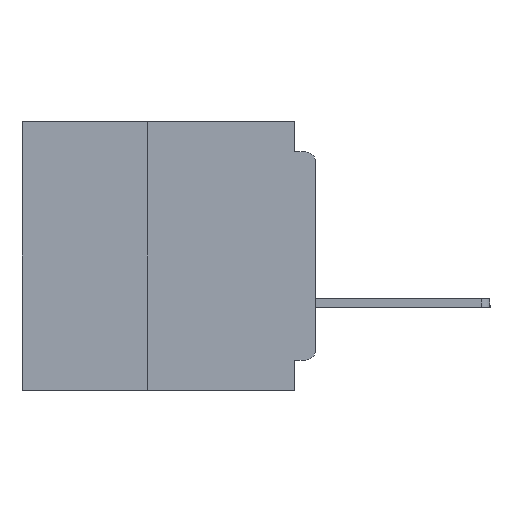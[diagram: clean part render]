
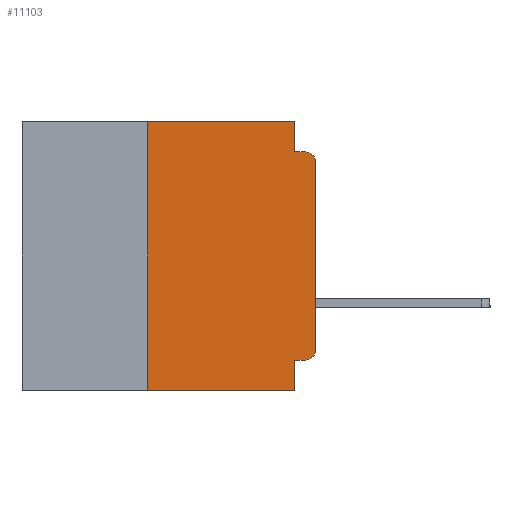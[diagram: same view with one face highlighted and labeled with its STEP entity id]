
A CAD part, left-side view. The second image highlights one B-rep face of the part: STEP entity #11103.
In plain terms, the highlighted planar face has unit normal (-1, 0, 0).
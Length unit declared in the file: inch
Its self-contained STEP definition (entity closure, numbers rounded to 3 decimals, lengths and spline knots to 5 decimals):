
#65 = CARTESIAN_POINT ( 'NONE',  ( 0., 0.031, -0.4 ) ) ;
#816 = AXIS2_PLACEMENT_3D ( 'NONE', #25689, #5339, #28968 ) ;
#1196 = EDGE_CURVE ( 'NONE', #15141, #7626, #9564, .T. ) ;
#1341 = VECTOR ( 'NONE', #21800, 39.37008 ) ;
#3353 = CIRCLE ( 'NONE', #23624, 0.015 ) ;
#3932 = VERTEX_POINT ( 'NONE', #65 ) ;
#4662 = CARTESIAN_POINT ( 'NONE',  ( 0., 0.25, -0.4 ) ) ;
#4825 = FACE_OUTER_BOUND ( 'NONE', #36976, .T. ) ;
#5259 = CARTESIAN_POINT ( 'NONE',  ( 0., 0., 0. ) ) ;
#5339 = DIRECTION ( 'NONE',  ( 1., 0., 0. ) ) ;
#5525 = VECTOR ( 'NONE', #8779, 39.37008 ) ;
#5892 = DIRECTION ( 'NONE',  ( 0., 0., -1. ) ) ;
#6065 = CARTESIAN_POINT ( 'NONE',  ( 0., 0.015, -0.355 ) ) ;
#7496 = CARTESIAN_POINT ( 'NONE',  ( 0., 0.437, 0. ) ) ;
#7626 = VERTEX_POINT ( 'NONE', #27727 ) ;
#8749 = DIRECTION ( 'NONE',  ( 0., 0., 1. ) ) ;
#8779 = DIRECTION ( 'NONE',  ( 0., 0., 1. ) ) ;
#8889 = EDGE_CURVE ( 'NONE', #15141, #21092, #3353, .T. ) ;
#9010 = VERTEX_POINT ( 'NONE', #21100 ) ;
#9564 = LINE ( 'NONE', #28296, #35123 ) ;
#10329 = VERTEX_POINT ( 'NONE', #4662 ) ;
#10991 = DIRECTION ( 'NONE',  ( 0., -1., 0. ) ) ;
#11103 = ADVANCED_FACE ( 'NONE', ( #4825 ), #35420, .F. ) ;
#11639 = LINE ( 'NONE', #5259, #19604 ) ;
#12084 = ORIENTED_EDGE ( 'NONE', *, *, #42866, .F. ) ;
#12362 = CARTESIAN_POINT ( 'NONE',  ( 0., 0., -0.06 ) ) ;
#13687 = EDGE_CURVE ( 'NONE', #32011, #25730, #17010, .T. ) ;
#13967 = EDGE_CURVE ( 'NONE', #28992, #9010, #31956, .T. ) ;
#14778 = LINE ( 'NONE', #28915, #5525 ) ;
#14803 = EDGE_CURVE ( 'NONE', #10329, #3932, #32591, .T. ) ;
#15141 = VERTEX_POINT ( 'NONE', #6065 ) ;
#16264 = DIRECTION ( 'NONE',  ( -1., 0., 0. ) ) ;
#16553 = ORIENTED_EDGE ( 'NONE', *, *, #36174, .F. ) ;
#16655 = CARTESIAN_POINT ( 'NONE',  ( 0., 0.031, -0.045 ) ) ;
#17010 = CIRCLE ( 'NONE', #21538, 0.015 ) ;
#17339 = DIRECTION ( 'NONE',  ( 0., 0., -1. ) ) ;
#19075 = ORIENTED_EDGE ( 'NONE', *, *, #1196, .F. ) ;
#19317 = ORIENTED_EDGE ( 'NONE', *, *, #13967, .F. ) ;
#19604 = VECTOR ( 'NONE', #8749, 39.37008 ) ;
#20517 = DIRECTION ( 'NONE',  ( -1., 0., 0. ) ) ;
#21092 = VERTEX_POINT ( 'NONE', #27972 ) ;
#21100 = CARTESIAN_POINT ( 'NONE',  ( 0., 0.031, 0. ) ) ;
#21538 = AXIS2_PLACEMENT_3D ( 'NONE', #36018, #16264, #39305 ) ;
#21800 = DIRECTION ( 'NONE',  ( 0., -1., 0. ) ) ;
#22645 = ORIENTED_EDGE ( 'NONE', *, *, #14803, .T. ) ;
#23624 = AXIS2_PLACEMENT_3D ( 'NONE', #40164, #20517, #5892 ) ;
#23939 = EDGE_CURVE ( 'NONE', #21092, #32011, #11639, .T. ) ;
#24924 = VECTOR ( 'NONE', #37845, 39.37008 ) ;
#25301 = CARTESIAN_POINT ( 'NONE',  ( 0., 0.031, 0. ) ) ;
#25689 = CARTESIAN_POINT ( 'NONE',  ( 0., 0.437, 0. ) ) ;
#25730 = VERTEX_POINT ( 'NONE', #34843 ) ;
#26393 = VECTOR ( 'NONE', #17339, 39.37008 ) ;
#27727 = CARTESIAN_POINT ( 'NONE',  ( 0., 0.031, -0.355 ) ) ;
#27843 = ORIENTED_EDGE ( 'NONE', *, *, #23939, .T. ) ;
#27972 = CARTESIAN_POINT ( 'NONE',  ( 0., 0., -0.34 ) ) ;
#28243 = DIRECTION ( 'NONE',  ( 0., 1., 0. ) ) ;
#28296 = CARTESIAN_POINT ( 'NONE',  ( 0., 0., -0.355 ) ) ;
#28915 = CARTESIAN_POINT ( 'NONE',  ( 0., 0.25, -0.4 ) ) ;
#28968 = DIRECTION ( 'NONE',  ( 0., 0., -1. ) ) ;
#28992 = VERTEX_POINT ( 'NONE', #33139 ) ;
#29380 = LINE ( 'NONE', #38127, #1341 ) ;
#31891 = DIRECTION ( 'NONE',  ( 0., 0., -1. ) ) ;
#31956 = LINE ( 'NONE', #7496, #39621 ) ;
#32011 = VERTEX_POINT ( 'NONE', #12362 ) ;
#32591 = LINE ( 'NONE', #34548, #24924 ) ;
#33139 = CARTESIAN_POINT ( 'NONE',  ( 0., 0.25, 0. ) ) ;
#33728 = ORIENTED_EDGE ( 'NONE', *, *, #8889, .T. ) ;
#34548 = CARTESIAN_POINT ( 'NONE',  ( 0., 0.437, -0.4 ) ) ;
#34641 = VECTOR ( 'NONE', #31891, 39.37008 ) ;
#34843 = CARTESIAN_POINT ( 'NONE',  ( 0., 0.015, -0.045 ) ) ;
#35095 = LINE ( 'NONE', #40209, #26393 ) ;
#35123 = VECTOR ( 'NONE', #28243, 39.37008 ) ;
#35388 = EDGE_CURVE ( 'NONE', #7626, #3932, #35095, .T. ) ;
#35420 = PLANE ( 'NONE',  #816 ) ;
#36018 = CARTESIAN_POINT ( 'NONE',  ( 0., 0.015, -0.06 ) ) ;
#36174 = EDGE_CURVE ( 'NONE', #36517, #25730, #29380, .T. ) ;
#36517 = VERTEX_POINT ( 'NONE', #16655 ) ;
#36976 = EDGE_LOOP ( 'NONE', ( #27843, #41995, #16553, #42722, #19317, #12084, #22645, #39099, #19075, #33728 ) ) ;
#37845 = DIRECTION ( 'NONE',  ( 0., -1., 0. ) ) ;
#38127 = CARTESIAN_POINT ( 'NONE',  ( 0., 0., -0.045 ) ) ;
#39099 = ORIENTED_EDGE ( 'NONE', *, *, #35388, .F. ) ;
#39305 = DIRECTION ( 'NONE',  ( 0., 0., -1. ) ) ;
#39621 = VECTOR ( 'NONE', #10991, 39.37008 ) ;
#40082 = EDGE_CURVE ( 'NONE', #9010, #36517, #43296, .T. ) ;
#40164 = CARTESIAN_POINT ( 'NONE',  ( 0., 0.015, -0.34 ) ) ;
#40209 = CARTESIAN_POINT ( 'NONE',  ( 0., 0.031, -0.4 ) ) ;
#41995 = ORIENTED_EDGE ( 'NONE', *, *, #13687, .T. ) ;
#42722 = ORIENTED_EDGE ( 'NONE', *, *, #40082, .F. ) ;
#42866 = EDGE_CURVE ( 'NONE', #10329, #28992, #14778, .T. ) ;
#43296 = LINE ( 'NONE', #25301, #34641 ) ;
